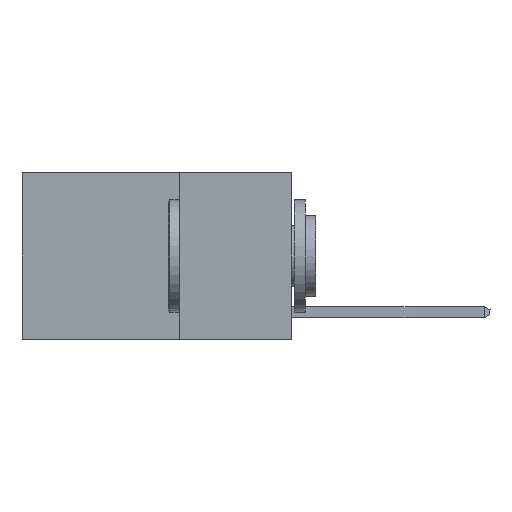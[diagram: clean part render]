
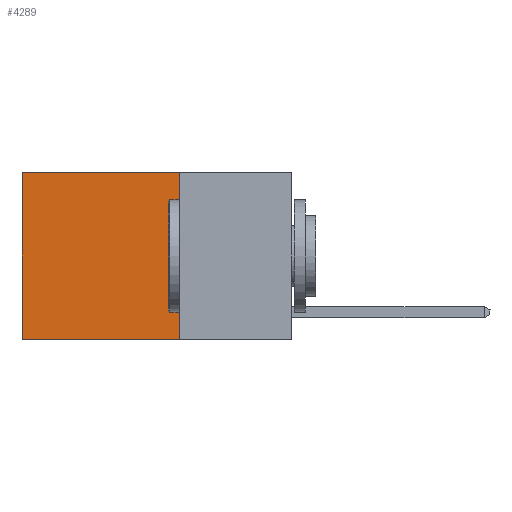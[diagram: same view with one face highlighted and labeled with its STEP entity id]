
A CAD part, left-side view. The second image highlights one B-rep face of the part: STEP entity #4289.
In plain terms, the highlighted planar face has unit normal (-1, 0, 0).
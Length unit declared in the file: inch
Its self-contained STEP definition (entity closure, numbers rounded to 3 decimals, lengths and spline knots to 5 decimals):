
#105 = EDGE_LOOP ( 'NONE', ( #26128, #1449, #4226, #28306 ) ) ;
#996 = VECTOR ( 'NONE', #10210, 39.37008 ) ;
#1220 = CARTESIAN_POINT ( 'NONE',  ( 0.2625, 0.25, -0.37 ) ) ;
#1449 = ORIENTED_EDGE ( 'NONE', *, *, #16222, .F. ) ;
#1502 = VERTEX_POINT ( 'NONE', #21413 ) ;
#2686 = EDGE_CURVE ( 'NONE', #30293, #21123, #19065, .T. ) ;
#4226 = ORIENTED_EDGE ( 'NONE', *, *, #25535, .F. ) ;
#4289 = ADVANCED_FACE ( 'NONE', ( #7660 ), #26384, .F. ) ;
#7660 = FACE_OUTER_BOUND ( 'NONE', #105, .T. ) ;
#7745 = CARTESIAN_POINT ( 'NONE',  ( 0.2625, 0.25, 0. ) ) ;
#8163 = CARTESIAN_POINT ( 'NONE',  ( 0.2625, 0.25, 0. ) ) ;
#8466 = DIRECTION ( 'NONE',  ( 0., 0., -1. ) ) ;
#10210 = DIRECTION ( 'NONE',  ( 0., 1., 0. ) ) ;
#14999 = CARTESIAN_POINT ( 'NONE',  ( 0.2625, 0.25, 0. ) ) ;
#16222 = EDGE_CURVE ( 'NONE', #1502, #21123, #20246, .T. ) ;
#17325 = CARTESIAN_POINT ( 'NONE',  ( 0.2625, 0.6, -0.37 ) ) ;
#18074 = DIRECTION ( 'NONE',  ( 0., 1., 0. ) ) ;
#18957 = DIRECTION ( 'NONE',  ( 0., 0., -1. ) ) ;
#19065 = LINE ( 'NONE', #23268, #25161 ) ;
#20246 = LINE ( 'NONE', #1220, #28470 ) ;
#20609 = AXIS2_PLACEMENT_3D ( 'NONE', #23768, #24069, #18957 ) ;
#21123 = VERTEX_POINT ( 'NONE', #17325 ) ;
#21413 = CARTESIAN_POINT ( 'NONE',  ( 0.2625, 0.25, -0.37 ) ) ;
#23268 = CARTESIAN_POINT ( 'NONE',  ( 0.2625, 0.6, 0. ) ) ;
#23768 = CARTESIAN_POINT ( 'NONE',  ( 0.2625, 0.25, 0. ) ) ;
#24069 = DIRECTION ( 'NONE',  ( 1., 0., 0. ) ) ;
#24840 = EDGE_CURVE ( 'NONE', #27176, #30293, #26628, .T. ) ;
#25161 = VECTOR ( 'NONE', #25741, 39.37008 ) ;
#25535 = EDGE_CURVE ( 'NONE', #27176, #1502, #29369, .T. ) ;
#25741 = DIRECTION ( 'NONE',  ( 0., 0., -1. ) ) ;
#26128 = ORIENTED_EDGE ( 'NONE', *, *, #2686, .T. ) ;
#26224 = VECTOR ( 'NONE', #8466, 39.37008 ) ;
#26384 = PLANE ( 'NONE',  #20609 ) ;
#26628 = LINE ( 'NONE', #14999, #996 ) ;
#27176 = VERTEX_POINT ( 'NONE', #7745 ) ;
#28306 = ORIENTED_EDGE ( 'NONE', *, *, #24840, .T. ) ;
#28470 = VECTOR ( 'NONE', #18074, 39.37008 ) ;
#29369 = LINE ( 'NONE', #8163, #26224 ) ;
#29833 = CARTESIAN_POINT ( 'NONE',  ( 0.2625, 0.6, 0. ) ) ;
#30293 = VERTEX_POINT ( 'NONE', #29833 ) ;
